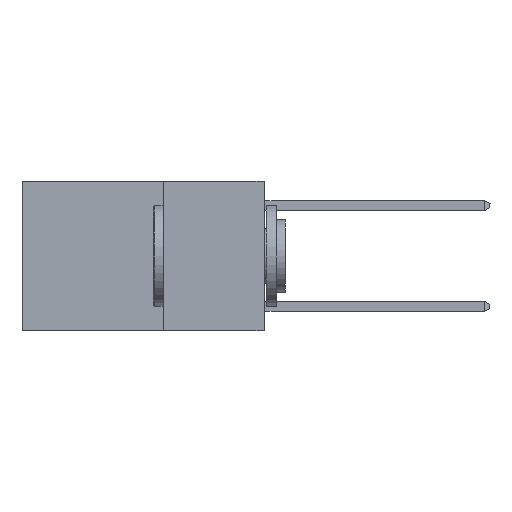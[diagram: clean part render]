
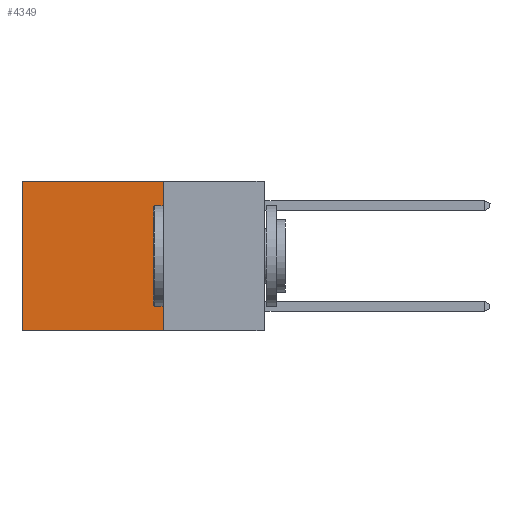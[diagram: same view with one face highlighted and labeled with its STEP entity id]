
A CAD part, left-side view. The second image highlights one B-rep face of the part: STEP entity #4349.
In plain terms, the highlighted planar face has unit normal (-1, 0, 0).
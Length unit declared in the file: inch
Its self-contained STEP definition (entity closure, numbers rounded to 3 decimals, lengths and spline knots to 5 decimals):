
#619 = VECTOR ( 'NONE', #24519, 39.37008 ) ;
#1023 = DIRECTION ( 'NONE',  ( 0., 0., -1. ) ) ;
#1344 = CARTESIAN_POINT ( 'NONE',  ( 0.2625, 0.6, -0.37 ) ) ;
#2310 = PLANE ( 'NONE',  #27566 ) ;
#2809 = LINE ( 'NONE', #9783, #17986 ) ;
#4349 = ADVANCED_FACE ( 'NONE', ( #16258 ), #2310, .F. ) ;
#7353 = ORIENTED_EDGE ( 'NONE', *, *, #11573, .T. ) ;
#7944 = LINE ( 'NONE', #13995, #19860 ) ;
#8545 = CARTESIAN_POINT ( 'NONE',  ( 0.2625, 0.25, 0. ) ) ;
#9783 = CARTESIAN_POINT ( 'NONE',  ( 0.2625, 0.25, 0. ) ) ;
#10769 = EDGE_CURVE ( 'NONE', #28123, #20059, #17631, .T. ) ;
#10902 = ORIENTED_EDGE ( 'NONE', *, *, #17246, .F. ) ;
#11477 = ORIENTED_EDGE ( 'NONE', *, *, #10769, .F. ) ;
#11573 = EDGE_CURVE ( 'NONE', #17542, #20059, #23514, .T. ) ;
#11607 = DIRECTION ( 'NONE',  ( 0., 1., 0. ) ) ;
#12070 = DIRECTION ( 'NONE',  ( 0., 0., -1. ) ) ;
#12339 = EDGE_LOOP ( 'NONE', ( #7353, #11477, #10902, #14251 ) ) ;
#13995 = CARTESIAN_POINT ( 'NONE',  ( 0.2625, 0.25, 0. ) ) ;
#14251 = ORIENTED_EDGE ( 'NONE', *, *, #24559, .T. ) ;
#16258 = FACE_OUTER_BOUND ( 'NONE', #12339, .T. ) ;
#17246 = EDGE_CURVE ( 'NONE', #20026, #28123, #2809, .T. ) ;
#17542 = VERTEX_POINT ( 'NONE', #22039 ) ;
#17631 = LINE ( 'NONE', #19883, #619 ) ;
#17824 = DIRECTION ( 'NONE',  ( 0., 0., -1. ) ) ;
#17986 = VECTOR ( 'NONE', #1023, 39.37008 ) ;
#19860 = VECTOR ( 'NONE', #11607, 39.37008 ) ;
#19883 = CARTESIAN_POINT ( 'NONE',  ( 0.2625, 0.25, -0.37 ) ) ;
#20026 = VERTEX_POINT ( 'NONE', #8545 ) ;
#20059 = VERTEX_POINT ( 'NONE', #1344 ) ;
#21692 = CARTESIAN_POINT ( 'NONE',  ( 0.2625, 0.6, 0. ) ) ;
#21763 = CARTESIAN_POINT ( 'NONE',  ( 0.2625, 0.25, 0. ) ) ;
#22039 = CARTESIAN_POINT ( 'NONE',  ( 0.2625, 0.6, 0. ) ) ;
#23514 = LINE ( 'NONE', #21692, #28021 ) ;
#24118 = DIRECTION ( 'NONE',  ( 1., 0., 0. ) ) ;
#24519 = DIRECTION ( 'NONE',  ( 0., 1., 0. ) ) ;
#24559 = EDGE_CURVE ( 'NONE', #20026, #17542, #7944, .T. ) ;
#27512 = CARTESIAN_POINT ( 'NONE',  ( 0.2625, 0.25, -0.37 ) ) ;
#27566 = AXIS2_PLACEMENT_3D ( 'NONE', #21763, #24118, #12070 ) ;
#28021 = VECTOR ( 'NONE', #17824, 39.37008 ) ;
#28123 = VERTEX_POINT ( 'NONE', #27512 ) ;
